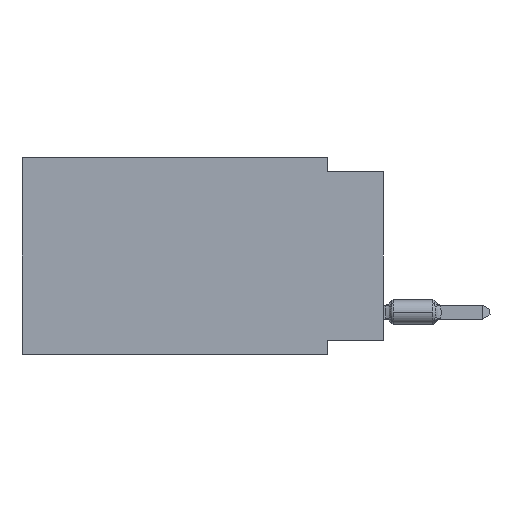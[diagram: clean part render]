
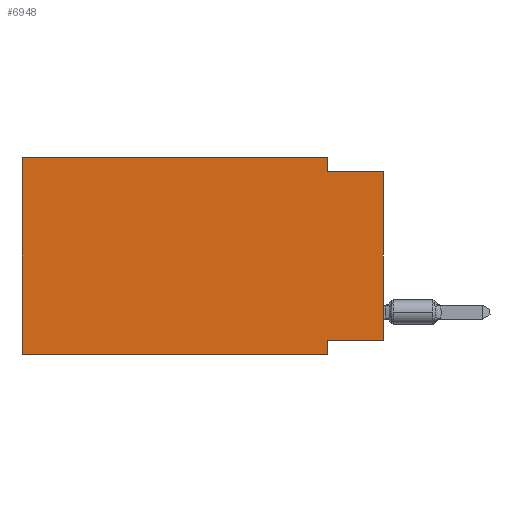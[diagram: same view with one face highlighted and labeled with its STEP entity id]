
A CAD part, left-side view. The second image highlights one B-rep face of the part: STEP entity #6948.
In plain terms, the highlighted planar face has unit normal (-1, 0, 0).
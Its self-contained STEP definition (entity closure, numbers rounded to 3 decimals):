
#43 = CARTESIAN_POINT ( 'NONE',  ( 0., 2.54, -8.89 ) ) ;
#137 = CARTESIAN_POINT ( 'NONE',  ( 0., 16.383, 0. ) ) ;
#343 = LINE ( 'NONE', #12470, #8959 ) ;
#538 = CARTESIAN_POINT ( 'NONE',  ( 0., 0., -8.255 ) ) ;
#875 = VERTEX_POINT ( 'NONE', #4569 ) ;
#1129 = VERTEX_POINT ( 'NONE', #9724 ) ;
#1478 = LINE ( 'NONE', #43, #10381 ) ;
#1561 = LINE ( 'NONE', #6724, #2104 ) ;
#1756 = LINE ( 'NONE', #137, #7845 ) ;
#1993 = EDGE_CURVE ( 'NONE', #4948, #4961, #10118, .T. ) ;
#2005 = DIRECTION ( 'NONE',  ( 0., 0., -1. ) ) ;
#2104 = VECTOR ( 'NONE', #2825, 1000. ) ;
#2629 = VECTOR ( 'NONE', #2005, 1000. ) ;
#2707 = LINE ( 'NONE', #13293, #13031 ) ;
#2825 = DIRECTION ( 'NONE',  ( 0., -1., 0. ) ) ;
#3124 = EDGE_CURVE ( 'NONE', #6732, #4961, #1478, .T. ) ;
#4374 = CARTESIAN_POINT ( 'NONE',  ( 0., 16.383, -8.89 ) ) ;
#4528 = ORIENTED_EDGE ( 'NONE', *, *, #3124, .F. ) ;
#4569 = CARTESIAN_POINT ( 'NONE',  ( 0., 16.383, 0. ) ) ;
#4811 = ORIENTED_EDGE ( 'NONE', *, *, #7468, .F. ) ;
#4948 = VERTEX_POINT ( 'NONE', #4374 ) ;
#4961 = VERTEX_POINT ( 'NONE', #9809 ) ;
#5449 = CARTESIAN_POINT ( 'NONE',  ( 0., 16.383, 0. ) ) ;
#5645 = DIRECTION ( 'NONE',  ( 0., 0., 1. ) ) ;
#6180 = EDGE_CURVE ( 'NONE', #4948, #875, #1756, .T. ) ;
#6558 = VERTEX_POINT ( 'NONE', #16572 ) ;
#6719 = ORIENTED_EDGE ( 'NONE', *, *, #10685, .F. ) ;
#6724 = CARTESIAN_POINT ( 'NONE',  ( 0., 0., -0.635 ) ) ;
#6732 = VERTEX_POINT ( 'NONE', #17006 ) ;
#6944 = VECTOR ( 'NONE', #9910, 1000. ) ;
#6948 = ADVANCED_FACE ( 'NONE', ( #9545 ), #9806, .F. ) ;
#7094 = LINE ( 'NONE', #12616, #6944 ) ;
#7387 = EDGE_LOOP ( 'NONE', ( #10886, #4811, #6719, #9915, #11532, #9472, #4528, #16170 ) ) ;
#7468 = EDGE_CURVE ( 'NONE', #16127, #6558, #1561, .T. ) ;
#7796 = EDGE_CURVE ( 'NONE', #16089, #6732, #343, .T. ) ;
#7845 = VECTOR ( 'NONE', #5645, 1000. ) ;
#8451 = DIRECTION ( 'NONE',  ( 0., 0., -1. ) ) ;
#8959 = VECTOR ( 'NONE', #9763, 1000. ) ;
#9472 = ORIENTED_EDGE ( 'NONE', *, *, #1993, .T. ) ;
#9545 = FACE_OUTER_BOUND ( 'NONE', #7387, .T. ) ;
#9724 = CARTESIAN_POINT ( 'NONE',  ( 0., 2.54, 0. ) ) ;
#9763 = DIRECTION ( 'NONE',  ( 0., 1., 0. ) ) ;
#9806 = PLANE ( 'NONE',  #13325 ) ;
#9809 = CARTESIAN_POINT ( 'NONE',  ( 0., 2.54, -8.89 ) ) ;
#9910 = DIRECTION ( 'NONE',  ( 0., -1., 0. ) ) ;
#9915 = ORIENTED_EDGE ( 'NONE', *, *, #17025, .F. ) ;
#10118 = LINE ( 'NONE', #16704, #10186 ) ;
#10186 = VECTOR ( 'NONE', #14277, 1000. ) ;
#10381 = VECTOR ( 'NONE', #8451, 1000. ) ;
#10388 = EDGE_CURVE ( 'NONE', #16089, #6558, #2707, .T. ) ;
#10685 = EDGE_CURVE ( 'NONE', #1129, #16127, #15931, .T. ) ;
#10886 = ORIENTED_EDGE ( 'NONE', *, *, #10388, .T. ) ;
#11532 = ORIENTED_EDGE ( 'NONE', *, *, #6180, .F. ) ;
#12470 = CARTESIAN_POINT ( 'NONE',  ( 0., 0., -8.255 ) ) ;
#12616 = CARTESIAN_POINT ( 'NONE',  ( 0., 16.383, 0. ) ) ;
#13031 = VECTOR ( 'NONE', #15523, 1000. ) ;
#13293 = CARTESIAN_POINT ( 'NONE',  ( 0., 0., 0. ) ) ;
#13325 = AXIS2_PLACEMENT_3D ( 'NONE', #5449, #16498, #15311 ) ;
#13410 = CARTESIAN_POINT ( 'NONE',  ( 0., 2.54, 0. ) ) ;
#14277 = DIRECTION ( 'NONE',  ( 0., -1., 0. ) ) ;
#15311 = DIRECTION ( 'NONE',  ( 0., 0., -1. ) ) ;
#15365 = CARTESIAN_POINT ( 'NONE',  ( 0., 2.54, -0.635 ) ) ;
#15523 = DIRECTION ( 'NONE',  ( 0., 0., 1. ) ) ;
#15931 = LINE ( 'NONE', #13410, #2629 ) ;
#16089 = VERTEX_POINT ( 'NONE', #538 ) ;
#16127 = VERTEX_POINT ( 'NONE', #15365 ) ;
#16170 = ORIENTED_EDGE ( 'NONE', *, *, #7796, .F. ) ;
#16498 = DIRECTION ( 'NONE',  ( 1., 0., 0. ) ) ;
#16572 = CARTESIAN_POINT ( 'NONE',  ( 0., 0., -0.635 ) ) ;
#16704 = CARTESIAN_POINT ( 'NONE',  ( 0., 16.383, -8.89 ) ) ;
#17006 = CARTESIAN_POINT ( 'NONE',  ( 0., 2.54, -8.255 ) ) ;
#17025 = EDGE_CURVE ( 'NONE', #875, #1129, #7094, .T. ) ;
